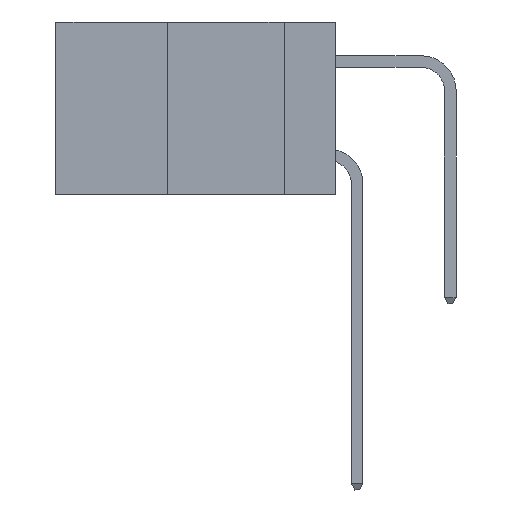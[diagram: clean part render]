
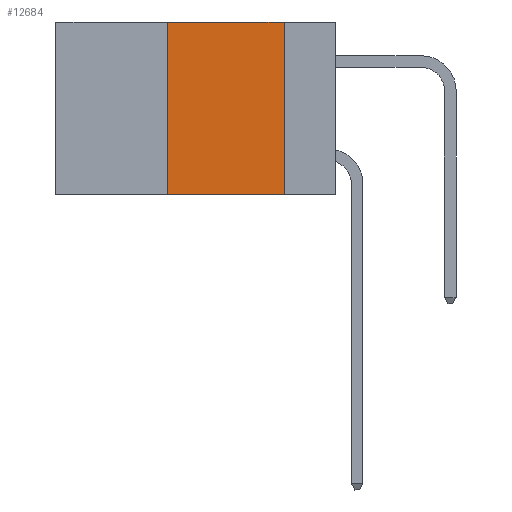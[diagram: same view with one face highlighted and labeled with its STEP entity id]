
A CAD part, left-side view. The second image highlights one B-rep face of the part: STEP entity #12684.
In plain terms, the highlighted planar face has unit normal (-1, 0, 0).
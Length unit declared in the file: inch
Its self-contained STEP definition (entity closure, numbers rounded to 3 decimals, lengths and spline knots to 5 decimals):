
#1845 = CARTESIAN_POINT ( 'NONE',  ( 0., 0.36, 0. ) ) ;
#2637 = DIRECTION ( 'NONE',  ( 0., 0., -1. ) ) ;
#4244 = LINE ( 'NONE', #22695, #10639 ) ;
#6442 = CARTESIAN_POINT ( 'NONE',  ( 0., 0.6, 0. ) ) ;
#8413 = EDGE_CURVE ( 'NONE', #21361, #13784, #29727, .T. ) ;
#9468 = CARTESIAN_POINT ( 'NONE',  ( 0., 0.11, -0.37 ) ) ;
#10605 = DIRECTION ( 'NONE',  ( 0., 0., -1. ) ) ;
#10639 = VECTOR ( 'NONE', #10605, 39.37008 ) ;
#11291 = DIRECTION ( 'NONE',  ( 0., -1., 0. ) ) ;
#11597 = VERTEX_POINT ( 'NONE', #9468 ) ;
#11646 = FACE_OUTER_BOUND ( 'NONE', #31367, .T. ) ;
#12246 = PLANE ( 'NONE',  #26347 ) ;
#12684 = ADVANCED_FACE ( 'NONE', ( #11646 ), #12246, .F. ) ;
#13784 = VERTEX_POINT ( 'NONE', #24227 ) ;
#14674 = CARTESIAN_POINT ( 'NONE',  ( 0., 0.6, 0. ) ) ;
#15035 = CARTESIAN_POINT ( 'NONE',  ( 0., 0.6, -0.37 ) ) ;
#17100 = DIRECTION ( 'NONE',  ( 1., 0., 0. ) ) ;
#17281 = CARTESIAN_POINT ( 'NONE',  ( 0., 0.36, -0.37 ) ) ;
#17362 = VERTEX_POINT ( 'NONE', #17281 ) ;
#21361 = VERTEX_POINT ( 'NONE', #29919 ) ;
#22254 = DIRECTION ( 'NONE',  ( 0., -1., 0. ) ) ;
#22695 = CARTESIAN_POINT ( 'NONE',  ( 0., 0.11, 0. ) ) ;
#23259 = VECTOR ( 'NONE', #11291, 39.37008 ) ;
#24227 = CARTESIAN_POINT ( 'NONE',  ( 0., 0.11, 0. ) ) ;
#24296 = VECTOR ( 'NONE', #31178, 39.37008 ) ;
#24401 = ORIENTED_EDGE ( 'NONE', *, *, #8413, .F. ) ;
#25211 = LINE ( 'NONE', #15035, #30873 ) ;
#25928 = EDGE_CURVE ( 'NONE', #13784, #11597, #4244, .T. ) ;
#26171 = ORIENTED_EDGE ( 'NONE', *, *, #28471, .T. ) ;
#26347 = AXIS2_PLACEMENT_3D ( 'NONE', #14674, #17100, #2637 ) ;
#26462 = EDGE_CURVE ( 'NONE', #17362, #21361, #28449, .T. ) ;
#27848 = ORIENTED_EDGE ( 'NONE', *, *, #26462, .F. ) ;
#28449 = LINE ( 'NONE', #1845, #24296 ) ;
#28471 = EDGE_CURVE ( 'NONE', #17362, #11597, #25211, .T. ) ;
#29727 = LINE ( 'NONE', #6442, #23259 ) ;
#29919 = CARTESIAN_POINT ( 'NONE',  ( 0., 0.36, 0. ) ) ;
#30839 = ORIENTED_EDGE ( 'NONE', *, *, #25928, .F. ) ;
#30873 = VECTOR ( 'NONE', #22254, 39.37008 ) ;
#31178 = DIRECTION ( 'NONE',  ( 0., 0., 1. ) ) ;
#31367 = EDGE_LOOP ( 'NONE', ( #30839, #24401, #27848, #26171 ) ) ;
